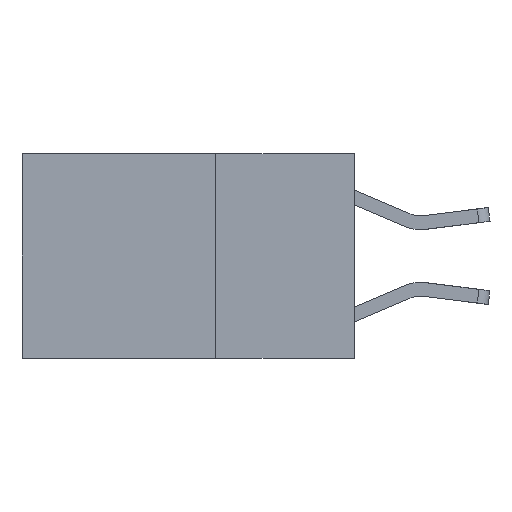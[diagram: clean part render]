
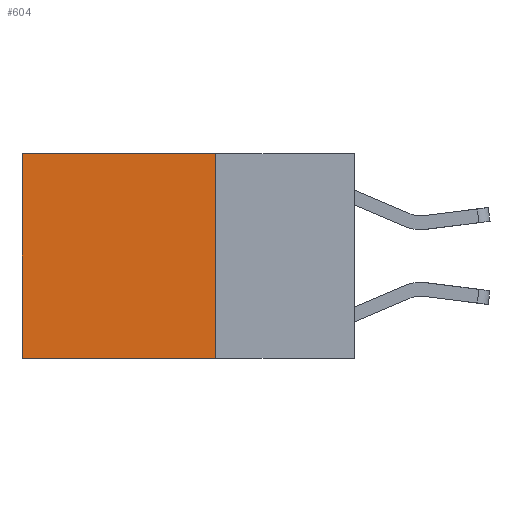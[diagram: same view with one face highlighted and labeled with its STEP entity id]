
A CAD part, left-side view. The second image highlights one B-rep face of the part: STEP entity #604.
In plain terms, the highlighted planar face has unit normal (-1, 0, 0).
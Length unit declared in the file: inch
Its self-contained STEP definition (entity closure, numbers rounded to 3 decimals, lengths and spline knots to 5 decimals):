
#354 = AXIS2_PLACEMENT_3D ( 'NONE', #6561, #3406, #4863 ) ;
#604 = ADVANCED_FACE ( 'NONE', ( #3227 ), #5882, .F. ) ;
#742 = EDGE_CURVE ( 'NONE', #5728, #8099, #5893, .T. ) ;
#812 = DIRECTION ( 'NONE',  ( 0., 1., 0. ) ) ;
#1315 = LINE ( 'NONE', #3563, #6836 ) ;
#1474 = CARTESIAN_POINT ( 'NONE',  ( 0.2625, 0.6, -0.37 ) ) ;
#1492 = LINE ( 'NONE', #3477, #5636 ) ;
#2220 = EDGE_CURVE ( 'NONE', #7158, #8099, #1315, .T. ) ;
#2746 = EDGE_CURVE ( 'NONE', #7250, #5728, #1492, .T. ) ;
#2979 = VECTOR ( 'NONE', #812, 39.37008 ) ;
#3030 = CARTESIAN_POINT ( 'NONE',  ( 0.2625, 0.25, -0.37 ) ) ;
#3227 = FACE_OUTER_BOUND ( 'NONE', #7780, .T. ) ;
#3406 = DIRECTION ( 'NONE',  ( 1., 0., 0. ) ) ;
#3477 = CARTESIAN_POINT ( 'NONE',  ( 0.2625, 0.25, 0. ) ) ;
#3501 = VECTOR ( 'NONE', #7647, 39.37008 ) ;
#3563 = CARTESIAN_POINT ( 'NONE',  ( 0.2625, 0.6, 0. ) ) ;
#4188 = ORIENTED_EDGE ( 'NONE', *, *, #2220, .T. ) ;
#4644 = ORIENTED_EDGE ( 'NONE', *, *, #2746, .F. ) ;
#4726 = CARTESIAN_POINT ( 'NONE',  ( 0.2625, 0.25, 0. ) ) ;
#4863 = DIRECTION ( 'NONE',  ( 0., 0., -1. ) ) ;
#4899 = EDGE_CURVE ( 'NONE', #7250, #7158, #5950, .T. ) ;
#5350 = DIRECTION ( 'NONE',  ( 0., 0., -1. ) ) ;
#5566 = CARTESIAN_POINT ( 'NONE',  ( 0.2625, 0.6, 0. ) ) ;
#5636 = VECTOR ( 'NONE', #5350, 39.37008 ) ;
#5728 = VERTEX_POINT ( 'NONE', #7937 ) ;
#5882 = PLANE ( 'NONE',  #354 ) ;
#5893 = LINE ( 'NONE', #3030, #3501 ) ;
#5950 = LINE ( 'NONE', #4726, #2979 ) ;
#6078 = DIRECTION ( 'NONE',  ( 0., 0., -1. ) ) ;
#6334 = CARTESIAN_POINT ( 'NONE',  ( 0.2625, 0.25, 0. ) ) ;
#6561 = CARTESIAN_POINT ( 'NONE',  ( 0.2625, 0.25, 0. ) ) ;
#6836 = VECTOR ( 'NONE', #6078, 39.37008 ) ;
#7158 = VERTEX_POINT ( 'NONE', #5566 ) ;
#7250 = VERTEX_POINT ( 'NONE', #6334 ) ;
#7288 = ORIENTED_EDGE ( 'NONE', *, *, #4899, .T. ) ;
#7647 = DIRECTION ( 'NONE',  ( 0., 1., 0. ) ) ;
#7780 = EDGE_LOOP ( 'NONE', ( #4188, #8122, #4644, #7288 ) ) ;
#7937 = CARTESIAN_POINT ( 'NONE',  ( 0.2625, 0.25, -0.37 ) ) ;
#8099 = VERTEX_POINT ( 'NONE', #1474 ) ;
#8122 = ORIENTED_EDGE ( 'NONE', *, *, #742, .F. ) ;
